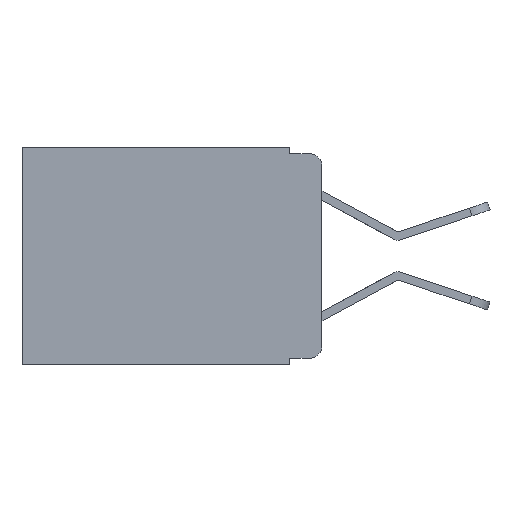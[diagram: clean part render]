
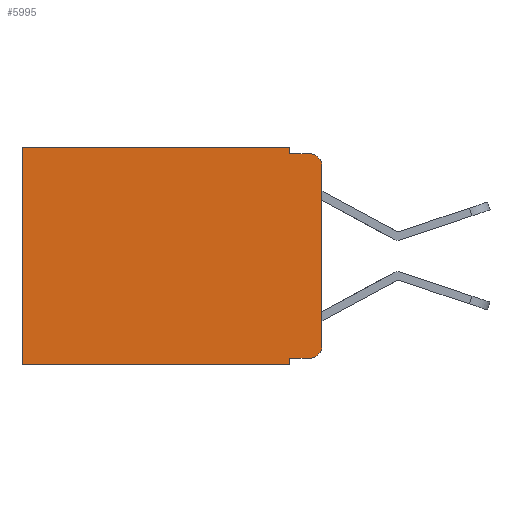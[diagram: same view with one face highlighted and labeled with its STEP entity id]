
A CAD part, left-side view. The second image highlights one B-rep face of the part: STEP entity #5995.
In plain terms, the highlighted planar face has unit normal (-1, 0, 0).
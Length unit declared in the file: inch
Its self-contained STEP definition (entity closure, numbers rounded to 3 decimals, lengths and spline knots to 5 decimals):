
#35 = CARTESIAN_POINT ( 'NONE',  ( 0.298, 0., -0.343 ) ) ;
#170 = EDGE_CURVE ( 'NONE', #3092, #3534, #9311, .T. ) ;
#180 = AXIS2_PLACEMENT_3D ( 'NONE', #5564, #4751, #8582 ) ;
#252 = EDGE_CURVE ( 'NONE', #446, #4117, #9788, .T. ) ;
#277 = EDGE_LOOP ( 'NONE', ( #8823, #6043, #8709, #337, #6118, #1662, #4127, #5551, #8840, #3737 ) ) ;
#337 = ORIENTED_EDGE ( 'NONE', *, *, #521, .F. ) ;
#344 = VECTOR ( 'NONE', #4032, 39.37008 ) ;
#446 = VERTEX_POINT ( 'NONE', #8294 ) ;
#521 = EDGE_CURVE ( 'NONE', #3092, #6547, #9205, .T. ) ;
#533 = VERTEX_POINT ( 'NONE', #3756 ) ;
#598 = DIRECTION ( 'NONE',  ( 1., 0., 0. ) ) ;
#808 = VECTOR ( 'NONE', #5278, 39.37008 ) ;
#1107 = CARTESIAN_POINT ( 'NONE',  ( 0.298, 0.473, 0. ) ) ;
#1292 = AXIS2_PLACEMENT_3D ( 'NONE', #5228, #598, #8454 ) ;
#1328 = LINE ( 'NONE', #1589, #3635 ) ;
#1489 = DIRECTION ( 'NONE',  ( 0., 0., -1. ) ) ;
#1589 = CARTESIAN_POINT ( 'NONE',  ( 0.298, 0.051, -0.333 ) ) ;
#1662 = ORIENTED_EDGE ( 'NONE', *, *, #5708, .T. ) ;
#1747 = VECTOR ( 'NONE', #5359, 39.37008 ) ;
#1938 = EDGE_CURVE ( 'NONE', #6547, #7412, #9679, .T. ) ;
#1958 = LINE ( 'NONE', #35, #8134 ) ;
#2265 = EDGE_CURVE ( 'NONE', #7797, #9795, #1958, .T. ) ;
#2748 = CARTESIAN_POINT ( 'NONE',  ( 0.298, 0., -0.313 ) ) ;
#2829 = CARTESIAN_POINT ( 'NONE',  ( 0.298, 0.051, 0. ) ) ;
#3004 = VECTOR ( 'NONE', #5221, 39.37008 ) ;
#3092 = VERTEX_POINT ( 'NONE', #6847 ) ;
#3534 = VERTEX_POINT ( 'NONE', #1107 ) ;
#3635 = VECTOR ( 'NONE', #3894, 39.37008 ) ;
#3677 = CARTESIAN_POINT ( 'NONE',  ( 0.298, 0.051, 0. ) ) ;
#3737 = ORIENTED_EDGE ( 'NONE', *, *, #252, .T. ) ;
#3756 = CARTESIAN_POINT ( 'NONE',  ( 0.298, 0.051, -0.333 ) ) ;
#3824 = CARTESIAN_POINT ( 'NONE',  ( 0.298, 0., 0. ) ) ;
#3877 = CARTESIAN_POINT ( 'NONE',  ( 0.298, 0.051, -0.01 ) ) ;
#3894 = DIRECTION ( 'NONE',  ( 0., -1., 0. ) ) ;
#4032 = DIRECTION ( 'NONE',  ( 0., 1., 0. ) ) ;
#4117 = VERTEX_POINT ( 'NONE', #2748 ) ;
#4127 = ORIENTED_EDGE ( 'NONE', *, *, #2265, .F. ) ;
#4344 = LINE ( 'NONE', #3677, #808 ) ;
#4358 = LINE ( 'NONE', #10047, #9219 ) ;
#4438 = DIRECTION ( 'NONE',  ( -1., 0., 0. ) ) ;
#4524 = PLANE ( 'NONE',  #1292 ) ;
#4673 = CARTESIAN_POINT ( 'NONE',  ( 0.298, 0.02, -0.01 ) ) ;
#4751 = DIRECTION ( 'NONE',  ( -1., 0., 0. ) ) ;
#5221 = DIRECTION ( 'NONE',  ( 0., 0., -1. ) ) ;
#5228 = CARTESIAN_POINT ( 'NONE',  ( 0.298, 0., 0. ) ) ;
#5278 = DIRECTION ( 'NONE',  ( 0., 0., -1. ) ) ;
#5359 = DIRECTION ( 'NONE',  ( 0., 0., -1. ) ) ;
#5551 = ORIENTED_EDGE ( 'NONE', *, *, #8887, .F. ) ;
#5564 = CARTESIAN_POINT ( 'NONE',  ( 0.298, 0.02, -0.313 ) ) ;
#5708 = EDGE_CURVE ( 'NONE', #3534, #9795, #5858, .T. ) ;
#5858 = LINE ( 'NONE', #8392, #1747 ) ;
#5995 = ADVANCED_FACE ( 'NONE', ( #7294 ), #4524, .F. ) ;
#6043 = ORIENTED_EDGE ( 'NONE', *, *, #6663, .T. ) ;
#6118 = ORIENTED_EDGE ( 'NONE', *, *, #170, .T. ) ;
#6360 = CARTESIAN_POINT ( 'NONE',  ( 0.298, 0.473, -0.343 ) ) ;
#6385 = AXIS2_PLACEMENT_3D ( 'NONE', #6655, #4438, #8336 ) ;
#6388 = CARTESIAN_POINT ( 'NONE',  ( 0.298, 0.051, -0.01 ) ) ;
#6547 = VERTEX_POINT ( 'NONE', #6388 ) ;
#6655 = CARTESIAN_POINT ( 'NONE',  ( 0.298, 0.02, -0.03 ) ) ;
#6663 = EDGE_CURVE ( 'NONE', #8879, #7412, #9256, .T. ) ;
#6847 = CARTESIAN_POINT ( 'NONE',  ( 0.298, 0.051, 0. ) ) ;
#6945 = DIRECTION ( 'NONE',  ( 0., -1., 0. ) ) ;
#7294 = FACE_OUTER_BOUND ( 'NONE', #277, .T. ) ;
#7412 = VERTEX_POINT ( 'NONE', #4673 ) ;
#7599 = CARTESIAN_POINT ( 'NONE',  ( 0.298, 0.051, -0.343 ) ) ;
#7780 = EDGE_CURVE ( 'NONE', #533, #446, #1328, .T. ) ;
#7797 = VERTEX_POINT ( 'NONE', #7599 ) ;
#8134 = VECTOR ( 'NONE', #9390, 39.37008 ) ;
#8294 = CARTESIAN_POINT ( 'NONE',  ( 0.298, 0.02, -0.333 ) ) ;
#8336 = DIRECTION ( 'NONE',  ( 0., 0., -1. ) ) ;
#8392 = CARTESIAN_POINT ( 'NONE',  ( 0.298, 0.473, 0. ) ) ;
#8454 = DIRECTION ( 'NONE',  ( 0., 0., -1. ) ) ;
#8492 = EDGE_CURVE ( 'NONE', #8879, #4117, #4358, .T. ) ;
#8582 = DIRECTION ( 'NONE',  ( 0., 0., -1. ) ) ;
#8709 = ORIENTED_EDGE ( 'NONE', *, *, #1938, .F. ) ;
#8823 = ORIENTED_EDGE ( 'NONE', *, *, #8492, .F. ) ;
#8840 = ORIENTED_EDGE ( 'NONE', *, *, #7780, .T. ) ;
#8879 = VERTEX_POINT ( 'NONE', #8976 ) ;
#8887 = EDGE_CURVE ( 'NONE', #533, #7797, #4344, .T. ) ;
#8976 = CARTESIAN_POINT ( 'NONE',  ( 0.298, 0., -0.03 ) ) ;
#9205 = LINE ( 'NONE', #2829, #3004 ) ;
#9219 = VECTOR ( 'NONE', #1489, 39.37008 ) ;
#9256 = CIRCLE ( 'NONE', #6385, 0.02 ) ;
#9311 = LINE ( 'NONE', #3824, #344 ) ;
#9390 = DIRECTION ( 'NONE',  ( 0., 1., 0. ) ) ;
#9679 = LINE ( 'NONE', #3877, #9922 ) ;
#9788 = CIRCLE ( 'NONE', #180, 0.02 ) ;
#9795 = VERTEX_POINT ( 'NONE', #6360 ) ;
#9922 = VECTOR ( 'NONE', #6945, 39.37008 ) ;
#10047 = CARTESIAN_POINT ( 'NONE',  ( 0.298, 0., 0. ) ) ;
